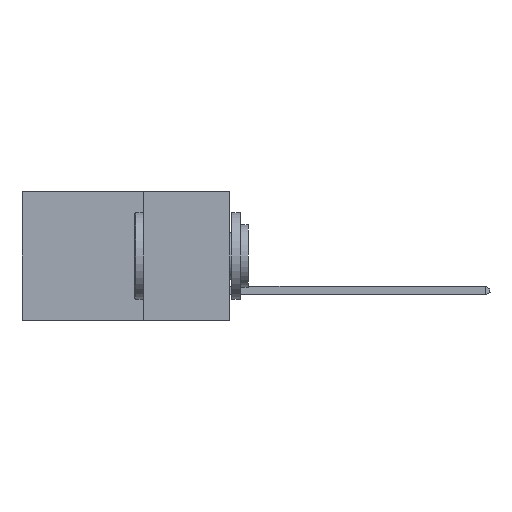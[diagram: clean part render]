
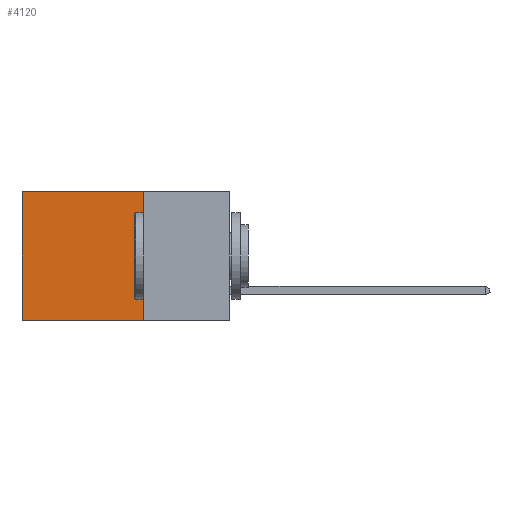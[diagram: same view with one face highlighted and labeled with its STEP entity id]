
A CAD part, left-side view. The second image highlights one B-rep face of the part: STEP entity #4120.
In plain terms, the highlighted planar face has unit normal (-1, 0, 0).
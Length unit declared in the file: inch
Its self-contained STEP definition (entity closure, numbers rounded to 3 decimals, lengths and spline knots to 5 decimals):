
#319 = VERTEX_POINT ( 'NONE', #5198 ) ;
#574 = LINE ( 'NONE', #16287, #26578 ) ;
#2748 = CARTESIAN_POINT ( 'NONE',  ( 0.298, 0.25, -0.37 ) ) ;
#3346 = CARTESIAN_POINT ( 'NONE',  ( 0.298, 0.25, 0. ) ) ;
#4120 = ADVANCED_FACE ( 'NONE', ( #19839 ), #10678, .F. ) ;
#4608 = EDGE_CURVE ( 'NONE', #18306, #22075, #574, .T. ) ;
#5104 = DIRECTION ( 'NONE',  ( 0., 0., -1. ) ) ;
#5198 = CARTESIAN_POINT ( 'NONE',  ( 0.298, 0.25, -0.37 ) ) ;
#7799 = DIRECTION ( 'NONE',  ( 0., 1., 0. ) ) ;
#8276 = LINE ( 'NONE', #27124, #12643 ) ;
#8632 = EDGE_LOOP ( 'NONE', ( #18638, #17253, #17381, #21771 ) ) ;
#10232 = LINE ( 'NONE', #14114, #24069 ) ;
#10491 = CARTESIAN_POINT ( 'NONE',  ( 0.298, 0.25, 0. ) ) ;
#10678 = PLANE ( 'NONE',  #18312 ) ;
#11245 = DIRECTION ( 'NONE',  ( 0., 1., 0. ) ) ;
#12584 = CARTESIAN_POINT ( 'NONE',  ( 0.298, 0.6, -0.37 ) ) ;
#12643 = VECTOR ( 'NONE', #5104, 39.37008 ) ;
#13726 = VECTOR ( 'NONE', #11245, 39.37008 ) ;
#14114 = CARTESIAN_POINT ( 'NONE',  ( 0.298, 0.6, 0. ) ) ;
#14770 = CARTESIAN_POINT ( 'NONE',  ( 0.298, 0.6, 0. ) ) ;
#16169 = DIRECTION ( 'NONE',  ( 0., 0., -1. ) ) ;
#16287 = CARTESIAN_POINT ( 'NONE',  ( 0.298, 0.25, 0. ) ) ;
#17253 = ORIENTED_EDGE ( 'NONE', *, *, #24756, .F. ) ;
#17381 = ORIENTED_EDGE ( 'NONE', *, *, #25802, .F. ) ;
#18306 = VERTEX_POINT ( 'NONE', #3346 ) ;
#18312 = AXIS2_PLACEMENT_3D ( 'NONE', #10491, #21621, #25963 ) ;
#18422 = LINE ( 'NONE', #2748, #13726 ) ;
#18638 = ORIENTED_EDGE ( 'NONE', *, *, #27222, .T. ) ;
#19839 = FACE_OUTER_BOUND ( 'NONE', #8632, .T. ) ;
#21621 = DIRECTION ( 'NONE',  ( 1., 0., 0. ) ) ;
#21771 = ORIENTED_EDGE ( 'NONE', *, *, #4608, .T. ) ;
#22075 = VERTEX_POINT ( 'NONE', #14770 ) ;
#22685 = VERTEX_POINT ( 'NONE', #12584 ) ;
#24069 = VECTOR ( 'NONE', #16169, 39.37008 ) ;
#24756 = EDGE_CURVE ( 'NONE', #319, #22685, #18422, .T. ) ;
#25802 = EDGE_CURVE ( 'NONE', #18306, #319, #8276, .T. ) ;
#25963 = DIRECTION ( 'NONE',  ( 0., 0., -1. ) ) ;
#26578 = VECTOR ( 'NONE', #7799, 39.37008 ) ;
#27124 = CARTESIAN_POINT ( 'NONE',  ( 0.298, 0.25, 0. ) ) ;
#27222 = EDGE_CURVE ( 'NONE', #22075, #22685, #10232, .T. ) ;
